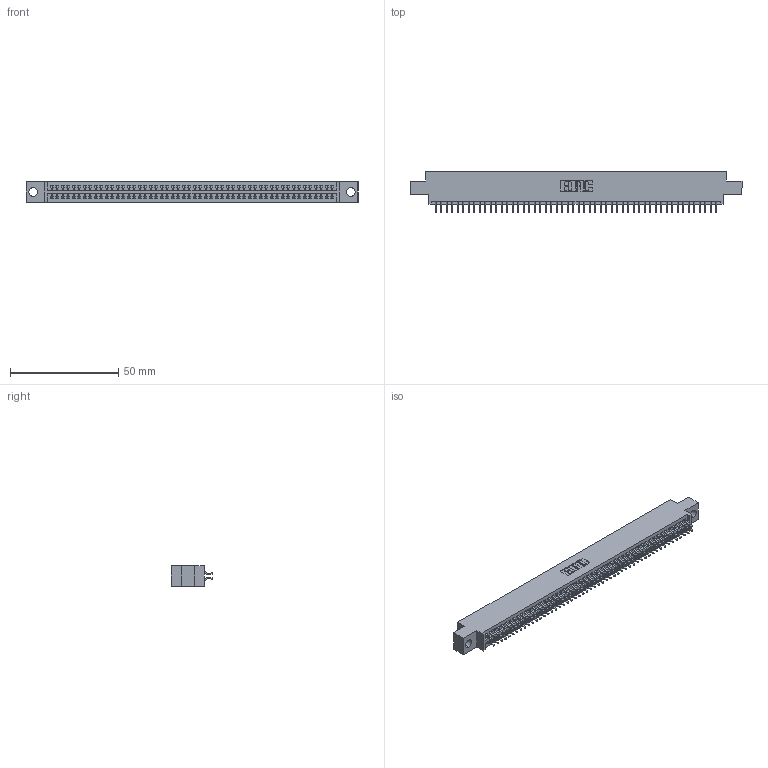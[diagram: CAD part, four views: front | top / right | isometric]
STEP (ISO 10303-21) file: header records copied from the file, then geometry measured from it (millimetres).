
FILE_DESCRIPTION (( 'STEP AP203' ), '1' );
FILE_NAME ('395-104-556-804.STEP', '2021-06-17T16:15:02', ( '' ), ( '' ), 'SwSTEP 2.0', 'SolidWorks 2020', '' );
FILE_SCHEMA (( 'CONFIG_CONTROL_DESIGN' ));
Length unit declared in the file: inch
Products named in the file (3): 345 Part_0.170 Offset - 0.156 Dia-TI; 345-292-001_556 Tail; 395-104-556-804
Assembly tree (105 placements, depth 2):
  395-104-556-804
    345 Part_0.170 Offset - 0.156 Dia-TI
    345-292-001_556 Tail  x104
Bounding box: 153.29 x 19.24 x 9.4 mm (x, y, z)
Volume: 14760 mm3; surface area: 21915.5 mm2
Topology: 105 solids, 105 shells, 5968 faces, 17757 edges, 11698 vertices
Faces by surface type: plane 3946, cylinder 2022
Entity records: 40225 total; most frequent: CARTESIAN_POINT 6754, ORIENTED_EDGE 6674, DIRECTION 5929, EDGE_CURVE 3337, VECTOR 2989, LINE 2989, VERTEX_POINT 2222, AXIS2_PLACEMENT_3D 1470
